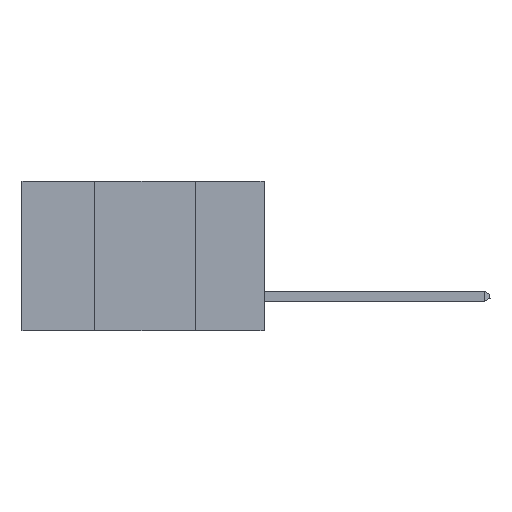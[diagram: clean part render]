
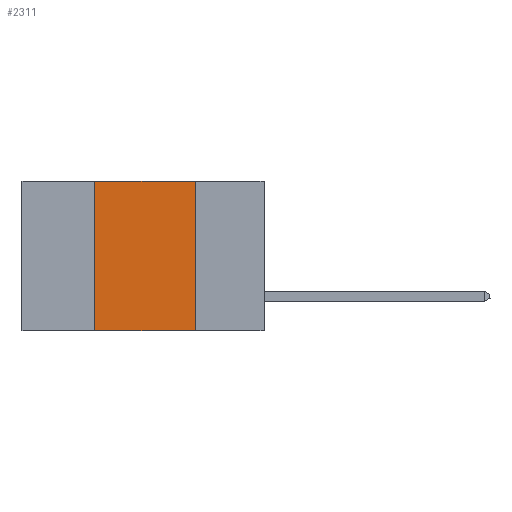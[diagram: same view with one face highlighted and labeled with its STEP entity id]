
A CAD part, left-side view. The second image highlights one B-rep face of the part: STEP entity #2311.
In plain terms, the highlighted planar face has unit normal (-1, 0, 0).
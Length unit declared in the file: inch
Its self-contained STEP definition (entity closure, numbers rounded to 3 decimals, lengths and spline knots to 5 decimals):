
#135 = ORIENTED_EDGE ( 'NONE', *, *, #7398, .F. ) ;
#484 = EDGE_CURVE ( 'NONE', #1640, #4657, #683, .T. ) ;
#542 = CARTESIAN_POINT ( 'NONE',  ( 0., 0.17, 0. ) ) ;
#587 = DIRECTION ( 'NONE',  ( 0., 0., -1. ) ) ;
#683 = LINE ( 'NONE', #3705, #2726 ) ;
#892 = EDGE_CURVE ( 'NONE', #1640, #3626, #7796, .T. ) ;
#1006 = EDGE_CURVE ( 'NONE', #5670, #4657, #1390, .T. ) ;
#1390 = LINE ( 'NONE', #542, #5388 ) ;
#1640 = VERTEX_POINT ( 'NONE', #8082 ) ;
#2311 = ADVANCED_FACE ( 'NONE', ( #3609 ), #3216, .F. ) ;
#2696 = CARTESIAN_POINT ( 'NONE',  ( 0., 0.17, 0. ) ) ;
#2726 = VECTOR ( 'NONE', #4822, 39.37008 ) ;
#3015 = AXIS2_PLACEMENT_3D ( 'NONE', #3152, #6196, #6185 ) ;
#3152 = CARTESIAN_POINT ( 'NONE',  ( 0., 0.6, 0. ) ) ;
#3216 = PLANE ( 'NONE',  #3015 ) ;
#3609 = FACE_OUTER_BOUND ( 'NONE', #9203, .T. ) ;
#3626 = VERTEX_POINT ( 'NONE', #9287 ) ;
#3705 = CARTESIAN_POINT ( 'NONE',  ( 0., 0.6, -0.37 ) ) ;
#4657 = VERTEX_POINT ( 'NONE', #7071 ) ;
#4770 = VECTOR ( 'NONE', #6715, 39.37008 ) ;
#4822 = DIRECTION ( 'NONE',  ( 0., -1., 0. ) ) ;
#5388 = VECTOR ( 'NONE', #587, 39.37008 ) ;
#5571 = ORIENTED_EDGE ( 'NONE', *, *, #1006, .F. ) ;
#5670 = VERTEX_POINT ( 'NONE', #2696 ) ;
#5724 = DIRECTION ( 'NONE',  ( 0., 0., 1. ) ) ;
#5975 = CARTESIAN_POINT ( 'NONE',  ( 0., 0.42, 0. ) ) ;
#6004 = VECTOR ( 'NONE', #5724, 39.37008 ) ;
#6185 = DIRECTION ( 'NONE',  ( 0., 0., -1. ) ) ;
#6196 = DIRECTION ( 'NONE',  ( 1., 0., 0. ) ) ;
#6715 = DIRECTION ( 'NONE',  ( 0., -1., 0. ) ) ;
#6778 = LINE ( 'NONE', #8005, #4770 ) ;
#7071 = CARTESIAN_POINT ( 'NONE',  ( 0., 0.17, -0.37 ) ) ;
#7398 = EDGE_CURVE ( 'NONE', #3626, #5670, #6778, .T. ) ;
#7796 = LINE ( 'NONE', #5975, #6004 ) ;
#8005 = CARTESIAN_POINT ( 'NONE',  ( 0., 0.6, 0. ) ) ;
#8070 = ORIENTED_EDGE ( 'NONE', *, *, #892, .F. ) ;
#8082 = CARTESIAN_POINT ( 'NONE',  ( 0., 0.42, -0.37 ) ) ;
#8246 = ORIENTED_EDGE ( 'NONE', *, *, #484, .T. ) ;
#9203 = EDGE_LOOP ( 'NONE', ( #5571, #135, #8070, #8246 ) ) ;
#9287 = CARTESIAN_POINT ( 'NONE',  ( 0., 0.42, 0. ) ) ;
